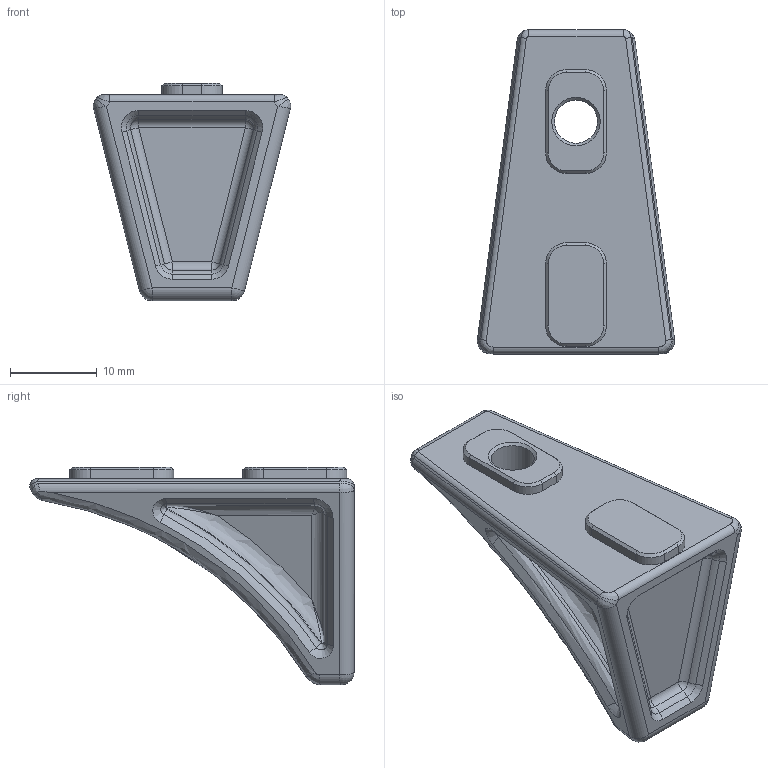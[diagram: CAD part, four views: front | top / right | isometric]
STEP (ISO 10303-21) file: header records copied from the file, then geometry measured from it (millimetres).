
FILE_DESCRIPTION(/* description */ (''),/* implementation_level */ '2;1');
FILE_NAME(/* name */ 'Standard.step',/* time_stamp */ '2021-06-02T00:24:39-04:00',/* author */ (''),/* organization */ (''),/* preprocessor_version */ 'ST-DEVELOPER v18.1',/* originating_system */ 'Autodesk Translation Framework v10.9.0.1377',/* authorisation */ '');
FILE_SCHEMA (('AUTOMOTIVE_DESIGN { 1 0 10303 214 3 1 1 }'));
Length unit declared in the file: millimetre
Products named in the file (1): Standard
Bounding box: 22.81 x 37.48 x 25.15 mm (x, y, z)
Volume: 5483.8 mm3; surface area: 2977.1 mm2
Topology: 1 solids, 1 shells, 156 faces, 349 edges, 191 vertices
Faces by surface type: bspline 44, cylinder 44, plane 41, cone 15, torus 6, sphere 6
Full cylindrical faces by diameter (mm): 5 x1, 9.3 x1
Entity records: 5803 total; most frequent: CARTESIAN_POINT 2553, ORIENTED_EDGE 678, DIRECTION 630, EDGE_CURVE 339, AXIS2_PLACEMENT_3D 241, VERTEX_POINT 191, EDGE_LOOP 164, FACE_OUTER_BOUND 156
